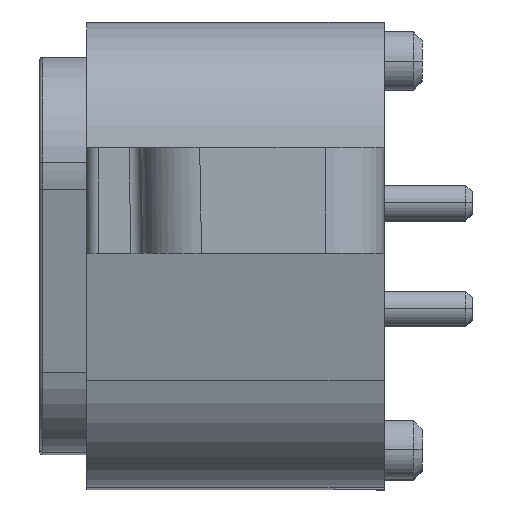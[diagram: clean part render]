
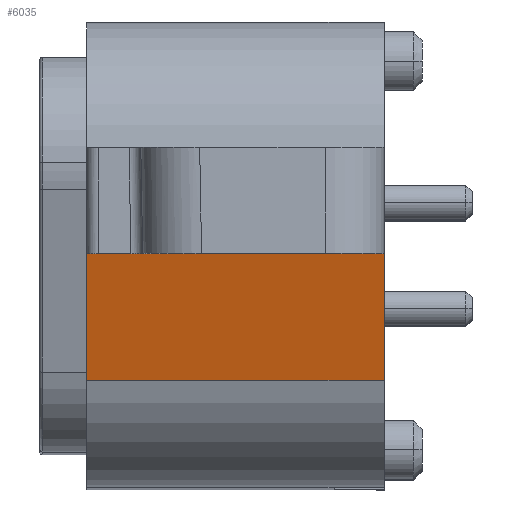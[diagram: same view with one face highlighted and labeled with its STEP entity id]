
A CAD part, top view. The second image highlights one B-rep face of the part: STEP entity #6035.
In plain terms, the highlighted planar face has unit normal (0, -0.241, 0.971).
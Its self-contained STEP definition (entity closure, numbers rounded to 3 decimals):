
#131 = EDGE_CURVE ( 'NONE', #3668, #9223, #9840, .T. ) ;
#319 = DIRECTION ( 'NONE',  ( -1., 0., 0. ) ) ;
#673 = VERTEX_POINT ( 'NONE', #2401 ) ;
#698 = CARTESIAN_POINT ( 'NONE',  ( -80.373, -7.525, 15.294 ) ) ;
#1015 = CARTESIAN_POINT ( 'NONE',  ( -85.423, -7.525, 15.294 ) ) ;
#1272 = PLANE ( 'NONE',  #7238 ) ;
#1668 = VECTOR ( 'NONE', #3240, 1000. ) ;
#1723 = ORIENTED_EDGE ( 'NONE', *, *, #6919, .F. ) ;
#2340 = ORIENTED_EDGE ( 'NONE', *, *, #10892, .F. ) ;
#2401 = CARTESIAN_POINT ( 'NONE',  ( -80.373, -9.675, 14.76 ) ) ;
#2411 = LINE ( 'NONE', #6338, #9343 ) ;
#3240 = DIRECTION ( 'NONE',  ( 1., 0., 0. ) ) ;
#3242 = CARTESIAN_POINT ( 'NONE',  ( -80.373, -7.525, 15.294 ) ) ;
#3668 = VERTEX_POINT ( 'NONE', #10763 ) ;
#3931 = ORIENTED_EDGE ( 'NONE', *, *, #131, .F. ) ;
#4623 = DIRECTION ( 'NONE',  ( 0., -0.971, -0.241 ) ) ;
#4864 = EDGE_CURVE ( 'NONE', #11237, #673, #8151, .T. ) ;
#4943 = DIRECTION ( 'NONE',  ( 1., 0., 0. ) ) ;
#5141 = VECTOR ( 'NONE', #4623, 1000. ) ;
#5214 = CARTESIAN_POINT ( 'NONE',  ( -82.898, -8.6, 15.027 ) ) ;
#6035 = ADVANCED_FACE ( 'NONE', ( #10095 ), #1272, .T. ) ;
#6338 = CARTESIAN_POINT ( 'NONE',  ( -85.423, -9.675, 14.76 ) ) ;
#6919 = EDGE_CURVE ( 'NONE', #11237, #3668, #2411, .T. ) ;
#7191 = ORIENTED_EDGE ( 'NONE', *, *, #4864, .T. ) ;
#7238 = AXIS2_PLACEMENT_3D ( 'NONE', #5214, #9140, #319 ) ;
#8151 = LINE ( 'NONE', #12050, #1668 ) ;
#8540 = CARTESIAN_POINT ( 'NONE',  ( -85.423, -9.675, 14.76 ) ) ;
#9140 = DIRECTION ( 'NONE',  ( 0., -0.241, 0.971 ) ) ;
#9223 = VERTEX_POINT ( 'NONE', #3242 ) ;
#9343 = VECTOR ( 'NONE', #10253, 1000. ) ;
#9532 = LINE ( 'NONE', #698, #5141 ) ;
#9840 = LINE ( 'NONE', #1015, #11857 ) ;
#10095 = FACE_OUTER_BOUND ( 'NONE', #12604, .T. ) ;
#10253 = DIRECTION ( 'NONE',  ( 0., 0.971, 0.241 ) ) ;
#10763 = CARTESIAN_POINT ( 'NONE',  ( -85.423, -7.525, 15.294 ) ) ;
#10892 = EDGE_CURVE ( 'NONE', #9223, #673, #9532, .T. ) ;
#11237 = VERTEX_POINT ( 'NONE', #8540 ) ;
#11857 = VECTOR ( 'NONE', #4943, 1000. ) ;
#12050 = CARTESIAN_POINT ( 'NONE',  ( -85.423, -9.675, 14.76 ) ) ;
#12604 = EDGE_LOOP ( 'NONE', ( #1723, #7191, #2340, #3931 ) ) ;
